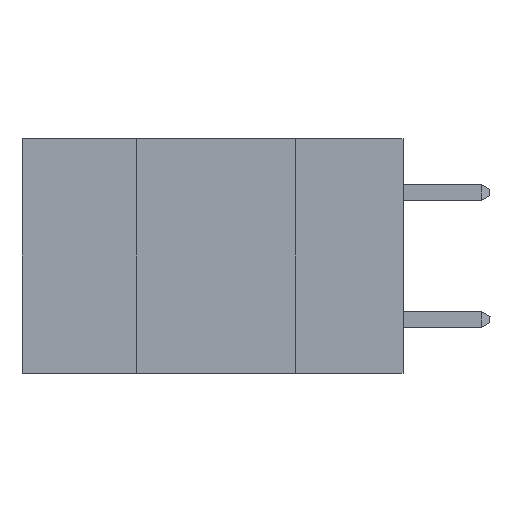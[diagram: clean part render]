
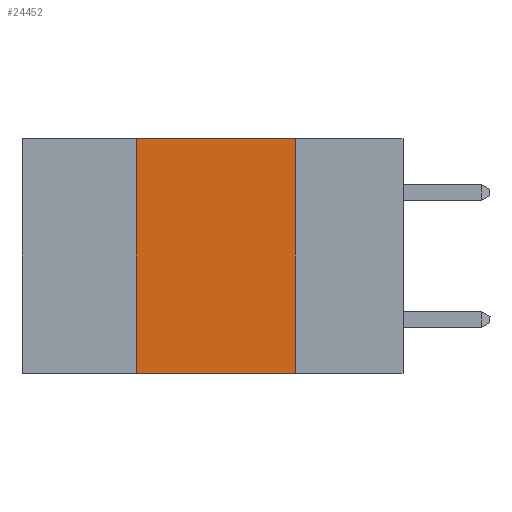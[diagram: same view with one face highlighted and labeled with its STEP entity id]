
A CAD part, left-side view. The second image highlights one B-rep face of the part: STEP entity #24452.
In plain terms, the highlighted planar face has unit normal (-1, 0, 0).
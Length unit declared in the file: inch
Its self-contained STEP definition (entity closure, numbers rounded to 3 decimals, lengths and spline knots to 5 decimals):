
#892 = DIRECTION ( 'NONE',  ( 0., 0., -1. ) ) ;
#1120 = ORIENTED_EDGE ( 'NONE', *, *, #39425, .F. ) ;
#1329 = ORIENTED_EDGE ( 'NONE', *, *, #13741, .F. ) ;
#7893 = AXIS2_PLACEMENT_3D ( 'NONE', #8427, #22084, #892 ) ;
#8427 = CARTESIAN_POINT ( 'NONE',  ( 0., 0.6, 0. ) ) ;
#9897 = VERTEX_POINT ( 'NONE', #19078 ) ;
#10782 = CARTESIAN_POINT ( 'NONE',  ( 0., 0.6, -0.37 ) ) ;
#12421 = VECTOR ( 'NONE', #26930, 39.37008 ) ;
#13741 = EDGE_CURVE ( 'NONE', #15603, #45678, #15632, .T. ) ;
#14943 = ORIENTED_EDGE ( 'NONE', *, *, #29803, .F. ) ;
#15603 = VERTEX_POINT ( 'NONE', #15666 ) ;
#15632 = LINE ( 'NONE', #30003, #12421 ) ;
#15666 = CARTESIAN_POINT ( 'NONE',  ( 0., 0.17, 0. ) ) ;
#15843 = EDGE_LOOP ( 'NONE', ( #1329, #1120, #14943, #43289 ) ) ;
#18318 = DIRECTION ( 'NONE',  ( 0., -1., 0. ) ) ;
#18641 = VECTOR ( 'NONE', #41522, 39.37008 ) ;
#19078 = CARTESIAN_POINT ( 'NONE',  ( 0., 0.42, -0.37 ) ) ;
#21379 = LINE ( 'NONE', #10782, #38519 ) ;
#21423 = VERTEX_POINT ( 'NONE', #34390 ) ;
#22084 = DIRECTION ( 'NONE',  ( 1., 0., 0. ) ) ;
#23371 = CARTESIAN_POINT ( 'NONE',  ( 0., 0.42, 0. ) ) ;
#24452 = ADVANCED_FACE ( 'NONE', ( #25633 ), #40019, .F. ) ;
#25633 = FACE_OUTER_BOUND ( 'NONE', #15843, .T. ) ;
#25927 = DIRECTION ( 'NONE',  ( 0., -1., 0. ) ) ;
#26156 = CARTESIAN_POINT ( 'NONE',  ( 0., 0.6, 0. ) ) ;
#26930 = DIRECTION ( 'NONE',  ( 0., 0., -1. ) ) ;
#29803 = EDGE_CURVE ( 'NONE', #9897, #21423, #38212, .T. ) ;
#29944 = CARTESIAN_POINT ( 'NONE',  ( 0., 0.17, -0.37 ) ) ;
#30003 = CARTESIAN_POINT ( 'NONE',  ( 0., 0.17, 0. ) ) ;
#30719 = VECTOR ( 'NONE', #25927, 39.37008 ) ;
#34390 = CARTESIAN_POINT ( 'NONE',  ( 0., 0.42, 0. ) ) ;
#36508 = EDGE_CURVE ( 'NONE', #9897, #45678, #21379, .T. ) ;
#38212 = LINE ( 'NONE', #23371, #18641 ) ;
#38519 = VECTOR ( 'NONE', #18318, 39.37008 ) ;
#39425 = EDGE_CURVE ( 'NONE', #21423, #15603, #40773, .T. ) ;
#40019 = PLANE ( 'NONE',  #7893 ) ;
#40773 = LINE ( 'NONE', #26156, #30719 ) ;
#41522 = DIRECTION ( 'NONE',  ( 0., 0., 1. ) ) ;
#43289 = ORIENTED_EDGE ( 'NONE', *, *, #36508, .T. ) ;
#45678 = VERTEX_POINT ( 'NONE', #29944 ) ;
